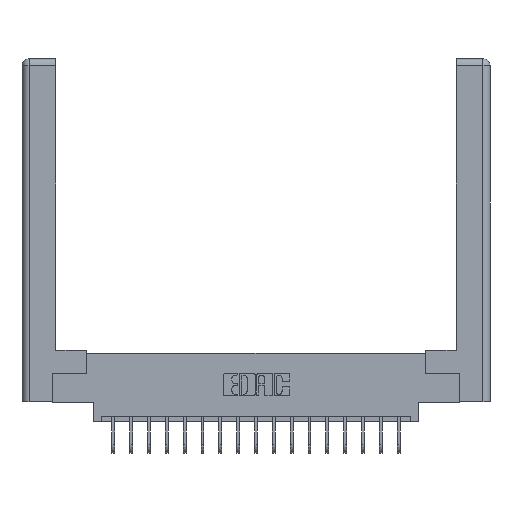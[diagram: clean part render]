
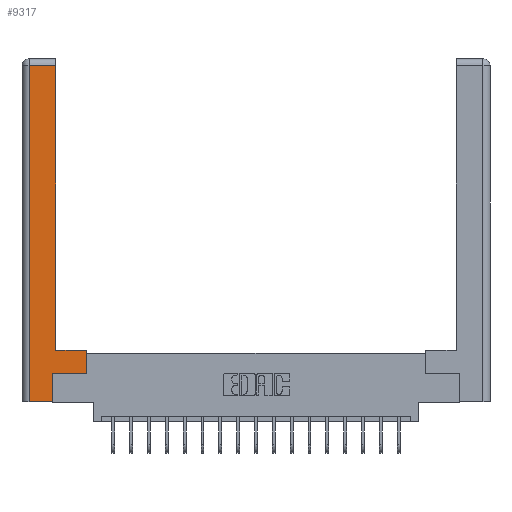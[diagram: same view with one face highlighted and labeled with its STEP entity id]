
A CAD part, top view. The second image highlights one B-rep face of the part: STEP entity #9317.
In plain terms, the highlighted planar face has unit normal (0, 0, 1).
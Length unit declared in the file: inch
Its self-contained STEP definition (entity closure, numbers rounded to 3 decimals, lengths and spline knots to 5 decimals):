
#242 = CARTESIAN_POINT ( 'NONE',  ( 0.565, 0.245, 0. ) ) ;
#355 = LINE ( 'NONE', #4137, #12131 ) ;
#1272 = ORIENTED_EDGE ( 'NONE', *, *, #2539, .T. ) ;
#1314 = ORIENTED_EDGE ( 'NONE', *, *, #11503, .T. ) ;
#1536 = DIRECTION ( 'NONE',  ( 1., 0., 0. ) ) ;
#1543 = VECTOR ( 'NONE', #12047, 39.37008 ) ;
#2128 = CARTESIAN_POINT ( 'NONE',  ( 0.265, 0.245, 0. ) ) ;
#2205 = CARTESIAN_POINT ( 'NONE',  ( 0.0615, 2.94, 0. ) ) ;
#2539 = EDGE_CURVE ( 'NONE', #14867, #16144, #355, .T. ) ;
#2636 = CARTESIAN_POINT ( 'NONE',  ( 0.265, 0., 0. ) ) ;
#2865 = DIRECTION ( 'NONE',  ( 0., 1., 0. ) ) ;
#3027 = DIRECTION ( 'NONE',  ( -1., 0., 0. ) ) ;
#3029 = LINE ( 'NONE', #2128, #18015 ) ;
#3137 = VECTOR ( 'NONE', #3481, 39.37008 ) ;
#3347 = DIRECTION ( 'NONE',  ( 0., 1., 0. ) ) ;
#3436 = ORIENTED_EDGE ( 'NONE', *, *, #16797, .T. ) ;
#3481 = DIRECTION ( 'NONE',  ( 0., 1., 0. ) ) ;
#4137 = CARTESIAN_POINT ( 'NONE',  ( 0.295, 0.45, 0. ) ) ;
#4264 = CARTESIAN_POINT ( 'NONE',  ( 0.295, 0.45, 0. ) ) ;
#4315 = ORIENTED_EDGE ( 'NONE', *, *, #9913, .T. ) ;
#5680 = PLANE ( 'NONE',  #7034 ) ;
#6089 = VERTEX_POINT ( 'NONE', #13581 ) ;
#6690 = CARTESIAN_POINT ( 'NONE',  ( 0.295, 2.94, 0. ) ) ;
#7004 = CARTESIAN_POINT ( 'NONE',  ( 0.295, 3., 0. ) ) ;
#7034 = AXIS2_PLACEMENT_3D ( 'NONE', #7204, #15966, #3027 ) ;
#7197 = ORIENTED_EDGE ( 'NONE', *, *, #14097, .T. ) ;
#7204 = CARTESIAN_POINT ( 'NONE',  ( 0., 0., 0. ) ) ;
#7425 = VECTOR ( 'NONE', #12781, 39.37008 ) ;
#7662 = CARTESIAN_POINT ( 'NONE',  ( 0.565, 0.45, 0. ) ) ;
#7905 = DIRECTION ( 'NONE',  ( -1., 0., 0. ) ) ;
#7918 = VERTEX_POINT ( 'NONE', #15372 ) ;
#8524 = VECTOR ( 'NONE', #2865, 39.37008 ) ;
#8588 = EDGE_LOOP ( 'NONE', ( #4315, #17324, #7197, #3436, #1314, #14509, #15969, #1272 ) ) ;
#8694 = VERTEX_POINT ( 'NONE', #6690 ) ;
#9195 = LINE ( 'NONE', #242, #16920 ) ;
#9317 = ADVANCED_FACE ( 'NONE', ( #14478 ), #5680, .F. ) ;
#9506 = CARTESIAN_POINT ( 'NONE',  ( 0.265, 0., 0. ) ) ;
#9913 = EDGE_CURVE ( 'NONE', #16144, #8694, #11465, .T. ) ;
#10050 = EDGE_CURVE ( 'NONE', #7918, #17661, #9195, .T. ) ;
#10569 = CARTESIAN_POINT ( 'NONE',  ( 0.0615, 0., 0. ) ) ;
#10611 = LINE ( 'NONE', #10569, #1543 ) ;
#11465 = LINE ( 'NONE', #7004, #8524 ) ;
#11503 = EDGE_CURVE ( 'NONE', #12289, #7918, #3029, .T. ) ;
#12047 = DIRECTION ( 'NONE',  ( 0., -1., 0. ) ) ;
#12083 = CARTESIAN_POINT ( 'NONE',  ( 0.565, 0.45, 0. ) ) ;
#12131 = VECTOR ( 'NONE', #18574, 39.37008 ) ;
#12184 = LINE ( 'NONE', #2636, #7425 ) ;
#12289 = VERTEX_POINT ( 'NONE', #9506 ) ;
#12446 = VERTEX_POINT ( 'NONE', #18069 ) ;
#12781 = DIRECTION ( 'NONE',  ( 1., 0., 0. ) ) ;
#13508 = CARTESIAN_POINT ( 'NONE',  ( 0.565, 0.245, 0. ) ) ;
#13581 = CARTESIAN_POINT ( 'NONE',  ( 0.0615, 0., 0. ) ) ;
#14097 = EDGE_CURVE ( 'NONE', #12446, #6089, #10611, .T. ) ;
#14138 = EDGE_CURVE ( 'NONE', #17661, #14867, #17900, .T. ) ;
#14330 = EDGE_CURVE ( 'NONE', #8694, #12446, #15833, .T. ) ;
#14478 = FACE_OUTER_BOUND ( 'NONE', #8588, .T. ) ;
#14509 = ORIENTED_EDGE ( 'NONE', *, *, #10050, .T. ) ;
#14867 = VERTEX_POINT ( 'NONE', #12083 ) ;
#15372 = CARTESIAN_POINT ( 'NONE',  ( 0.265, 0.245, 0. ) ) ;
#15599 = VECTOR ( 'NONE', #7905, 39.37008 ) ;
#15833 = LINE ( 'NONE', #2205, #15599 ) ;
#15966 = DIRECTION ( 'NONE',  ( 0., 0., -1. ) ) ;
#15969 = ORIENTED_EDGE ( 'NONE', *, *, #14138, .T. ) ;
#16144 = VERTEX_POINT ( 'NONE', #4264 ) ;
#16797 = EDGE_CURVE ( 'NONE', #6089, #12289, #12184, .T. ) ;
#16920 = VECTOR ( 'NONE', #1536, 39.37008 ) ;
#17324 = ORIENTED_EDGE ( 'NONE', *, *, #14330, .T. ) ;
#17661 = VERTEX_POINT ( 'NONE', #13508 ) ;
#17900 = LINE ( 'NONE', #7662, #3137 ) ;
#18015 = VECTOR ( 'NONE', #3347, 39.37008 ) ;
#18069 = CARTESIAN_POINT ( 'NONE',  ( 0.0615, 2.94, 0. ) ) ;
#18574 = DIRECTION ( 'NONE',  ( -1., 0., 0. ) ) ;
